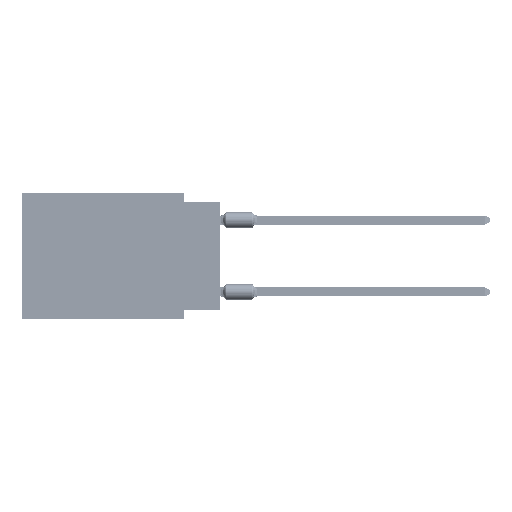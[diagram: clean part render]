
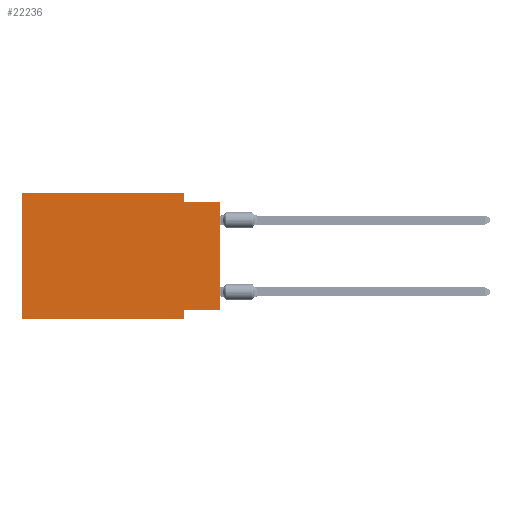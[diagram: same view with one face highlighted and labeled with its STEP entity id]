
A CAD part, left-side view. The second image highlights one B-rep face of the part: STEP entity #22236.
In plain terms, the highlighted planar face has unit normal (-1, 0, 0).
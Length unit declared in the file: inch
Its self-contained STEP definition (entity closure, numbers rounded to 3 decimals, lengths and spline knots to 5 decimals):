
#3340 = DIRECTION ( 'NONE',  ( 0., 0., -1. ) ) ;
#3929 = CARTESIAN_POINT ( 'NONE',  ( 0., 0.55, 0. ) ) ;
#5322 = EDGE_CURVE ( 'NONE', #67536, #30205, #65414, .T. ) ;
#5964 = EDGE_CURVE ( 'NONE', #30506, #42477, #24430, .T. ) ;
#8279 = EDGE_CURVE ( 'NONE', #42477, #70719, #61402, .T. ) ;
#10959 = DIRECTION ( 'NONE',  ( 1., 0., 0. ) ) ;
#11642 = AXIS2_PLACEMENT_3D ( 'NONE', #23707, #10959, #50089 ) ;
#14187 = CARTESIAN_POINT ( 'NONE',  ( 0., 0.1, 0. ) ) ;
#14757 = VECTOR ( 'NONE', #37100, 39.37008 ) ;
#16313 = DIRECTION ( 'NONE',  ( 0., 0., 1. ) ) ;
#17849 = CARTESIAN_POINT ( 'NONE',  ( 0., 0.1, 0. ) ) ;
#19703 = CARTESIAN_POINT ( 'NONE',  ( 0., 0.55, -0.35 ) ) ;
#20087 = ORIENTED_EDGE ( 'NONE', *, *, #73368, .T. ) ;
#20088 = LINE ( 'NONE', #20508, #73773 ) ;
#20508 = CARTESIAN_POINT ( 'NONE',  ( 0., 0., -0.325 ) ) ;
#21377 = CARTESIAN_POINT ( 'NONE',  ( 0., 0.1, -0.025 ) ) ;
#21894 = CARTESIAN_POINT ( 'NONE',  ( 0., 0.1, -0.35 ) ) ;
#22236 = ADVANCED_FACE ( 'NONE', ( #24934 ), #43514, .F. ) ;
#23707 = CARTESIAN_POINT ( 'NONE',  ( 0., 0.55, 0. ) ) ;
#23867 = CARTESIAN_POINT ( 'NONE',  ( 0., 0., -0.025 ) ) ;
#24430 = LINE ( 'NONE', #17849, #35372 ) ;
#24934 = FACE_OUTER_BOUND ( 'NONE', #69976, .T. ) ;
#25493 = LINE ( 'NONE', #19703, #14757 ) ;
#26063 = CARTESIAN_POINT ( 'NONE',  ( 0., 0.55, -0.35 ) ) ;
#27409 = VECTOR ( 'NONE', #41474, 39.37008 ) ;
#29065 = VECTOR ( 'NONE', #42044, 39.37008 ) ;
#30187 = EDGE_CURVE ( 'NONE', #30205, #30506, #34468, .T. ) ;
#30205 = VERTEX_POINT ( 'NONE', #79378 ) ;
#30299 = ORIENTED_EDGE ( 'NONE', *, *, #8279, .F. ) ;
#30506 = VERTEX_POINT ( 'NONE', #14187 ) ;
#31246 = CARTESIAN_POINT ( 'NONE',  ( 0., 0.1, -0.325 ) ) ;
#33949 = CARTESIAN_POINT ( 'NONE',  ( 0., 0., -0.325 ) ) ;
#34369 = EDGE_CURVE ( 'NONE', #40852, #67096, #20088, .T. ) ;
#34468 = LINE ( 'NONE', #47256, #76164 ) ;
#35028 = ORIENTED_EDGE ( 'NONE', *, *, #70293, .F. ) ;
#35372 = VECTOR ( 'NONE', #42613, 39.37008 ) ;
#35992 = ORIENTED_EDGE ( 'NONE', *, *, #5322, .F. ) ;
#37100 = DIRECTION ( 'NONE',  ( 0., -1., 0. ) ) ;
#38583 = EDGE_CURVE ( 'NONE', #67536, #56185, #25493, .T. ) ;
#40754 = VECTOR ( 'NONE', #3340, 39.37008 ) ;
#40852 = VERTEX_POINT ( 'NONE', #33949 ) ;
#41474 = DIRECTION ( 'NONE',  ( 0., 0., 1. ) ) ;
#42044 = DIRECTION ( 'NONE',  ( 0., -1., 0. ) ) ;
#42477 = VERTEX_POINT ( 'NONE', #21377 ) ;
#42613 = DIRECTION ( 'NONE',  ( 0., 0., -1. ) ) ;
#43514 = PLANE ( 'NONE',  #11642 ) ;
#43655 = VECTOR ( 'NONE', #16313, 39.37008 ) ;
#44849 = DIRECTION ( 'NONE',  ( 0., 1., 0. ) ) ;
#45013 = ORIENTED_EDGE ( 'NONE', *, *, #38583, .T. ) ;
#47256 = CARTESIAN_POINT ( 'NONE',  ( 0., 0.55, 0. ) ) ;
#47265 = LINE ( 'NONE', #65415, #43655 ) ;
#50089 = DIRECTION ( 'NONE',  ( 0., 0., -1. ) ) ;
#52313 = CARTESIAN_POINT ( 'NONE',  ( 0., 0., -0.025 ) ) ;
#55881 = ORIENTED_EDGE ( 'NONE', *, *, #5964, .F. ) ;
#56185 = VERTEX_POINT ( 'NONE', #69529 ) ;
#61402 = LINE ( 'NONE', #23867, #29065 ) ;
#65414 = LINE ( 'NONE', #3929, #27409 ) ;
#65415 = CARTESIAN_POINT ( 'NONE',  ( 0., 0., 0. ) ) ;
#66028 = LINE ( 'NONE', #21894, #40754 ) ;
#67096 = VERTEX_POINT ( 'NONE', #31246 ) ;
#67536 = VERTEX_POINT ( 'NONE', #26063 ) ;
#69529 = CARTESIAN_POINT ( 'NONE',  ( 0., 0.1, -0.35 ) ) ;
#69976 = EDGE_LOOP ( 'NONE', ( #20087, #30299, #55881, #74540, #35992, #45013, #35028, #74861 ) ) ;
#70293 = EDGE_CURVE ( 'NONE', #67096, #56185, #66028, .T. ) ;
#70719 = VERTEX_POINT ( 'NONE', #52313 ) ;
#73368 = EDGE_CURVE ( 'NONE', #40852, #70719, #47265, .T. ) ;
#73773 = VECTOR ( 'NONE', #44849, 39.37008 ) ;
#74540 = ORIENTED_EDGE ( 'NONE', *, *, #30187, .F. ) ;
#74861 = ORIENTED_EDGE ( 'NONE', *, *, #34369, .F. ) ;
#76164 = VECTOR ( 'NONE', #78172, 39.37008 ) ;
#78172 = DIRECTION ( 'NONE',  ( 0., -1., 0. ) ) ;
#79378 = CARTESIAN_POINT ( 'NONE',  ( 0., 0.55, 0. ) ) ;
